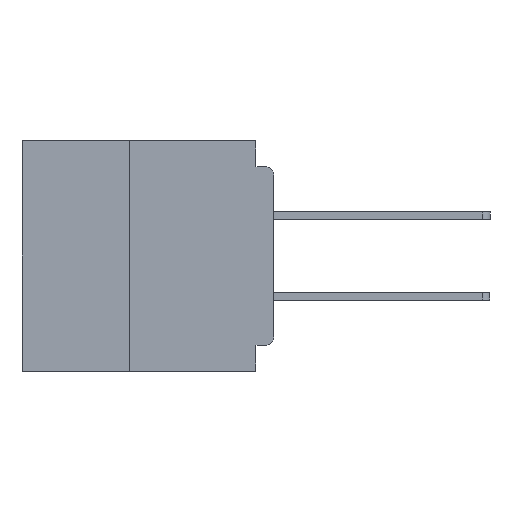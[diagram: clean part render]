
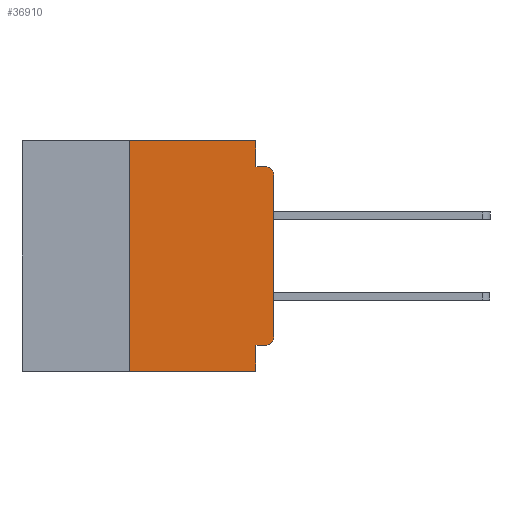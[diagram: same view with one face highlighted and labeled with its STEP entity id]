
A CAD part, left-side view. The second image highlights one B-rep face of the part: STEP entity #36910.
In plain terms, the highlighted planar face has unit normal (-1, 0, 0).
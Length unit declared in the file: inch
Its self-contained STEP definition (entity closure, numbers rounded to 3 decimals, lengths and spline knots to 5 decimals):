
#987 = CARTESIAN_POINT ( 'NONE',  ( 0., 0., -0.34 ) ) ;
#1331 = LINE ( 'NONE', #21667, #23645 ) ;
#1415 = EDGE_CURVE ( 'NONE', #28528, #23592, #11275, .T. ) ;
#1893 = ORIENTED_EDGE ( 'NONE', *, *, #25983, .F. ) ;
#2481 = VERTEX_POINT ( 'NONE', #31643 ) ;
#3035 = CARTESIAN_POINT ( 'NONE',  ( 0., 0., 0. ) ) ;
#3039 = CARTESIAN_POINT ( 'NONE',  ( 0., 0.25, -0.4 ) ) ;
#3169 = DIRECTION ( 'NONE',  ( 0., 0., 1. ) ) ;
#3193 = VECTOR ( 'NONE', #30604, 39.37008 ) ;
#3470 = EDGE_CURVE ( 'NONE', #35224, #23592, #12240, .T. ) ;
#3504 = CARTESIAN_POINT ( 'NONE',  ( 0., 0.015, -0.045 ) ) ;
#4850 = EDGE_CURVE ( 'NONE', #10057, #22910, #9841, .T. ) ;
#5433 = CARTESIAN_POINT ( 'NONE',  ( 0., 0.437, 0. ) ) ;
#5462 = EDGE_CURVE ( 'NONE', #35224, #2481, #33309, .T. ) ;
#6059 = DIRECTION ( 'NONE',  ( 0., 0., 1. ) ) ;
#7000 = CARTESIAN_POINT ( 'NONE',  ( 0., 0.437, -0.4 ) ) ;
#7153 = CARTESIAN_POINT ( 'NONE',  ( 0., 0.031, -0.4 ) ) ;
#7585 = LINE ( 'NONE', #32341, #38575 ) ;
#7809 = DIRECTION ( 'NONE',  ( -1., 0., 0. ) ) ;
#8521 = PLANE ( 'NONE',  #28601 ) ;
#9280 = VECTOR ( 'NONE', #3169, 39.37008 ) ;
#9346 = VECTOR ( 'NONE', #36983, 39.37008 ) ;
#9600 = CIRCLE ( 'NONE', #16299, 0.015 ) ;
#9841 = LINE ( 'NONE', #30610, #24982 ) ;
#9846 = DIRECTION ( 'NONE',  ( 0., -1., 0. ) ) ;
#10057 = VERTEX_POINT ( 'NONE', #24387 ) ;
#10333 = CARTESIAN_POINT ( 'NONE',  ( 0., 0.015, -0.355 ) ) ;
#11275 = LINE ( 'NONE', #13278, #3193 ) ;
#11592 = DIRECTION ( 'NONE',  ( 1., 0., 0. ) ) ;
#11731 = EDGE_CURVE ( 'NONE', #24256, #30757, #34052, .T. ) ;
#11870 = ORIENTED_EDGE ( 'NONE', *, *, #5462, .F. ) ;
#12240 = LINE ( 'NONE', #7000, #27360 ) ;
#13278 = CARTESIAN_POINT ( 'NONE',  ( 0., 0.031, -0.4 ) ) ;
#13606 = EDGE_CURVE ( 'NONE', #31149, #10057, #7585, .T. ) ;
#14590 = CARTESIAN_POINT ( 'NONE',  ( 0., 0.015, -0.34 ) ) ;
#15170 = ORIENTED_EDGE ( 'NONE', *, *, #4850, .F. ) ;
#15657 = ORIENTED_EDGE ( 'NONE', *, *, #11731, .T. ) ;
#16299 = AXIS2_PLACEMENT_3D ( 'NONE', #25949, #7809, #28965 ) ;
#17634 = DIRECTION ( 'NONE',  ( 0., 0., -1. ) ) ;
#18174 = VERTEX_POINT ( 'NONE', #38862 ) ;
#18314 = LINE ( 'NONE', #22138, #9346 ) ;
#18463 = FACE_OUTER_BOUND ( 'NONE', #36308, .T. ) ;
#19239 = VECTOR ( 'NONE', #6059, 39.37008 ) ;
#20994 = CARTESIAN_POINT ( 'NONE',  ( 0., 0.031, 0. ) ) ;
#21667 = CARTESIAN_POINT ( 'NONE',  ( 0., 0.437, 0. ) ) ;
#21884 = EDGE_CURVE ( 'NONE', #18174, #22910, #9600, .T. ) ;
#22124 = CARTESIAN_POINT ( 'NONE',  ( 0., 0.031, -0.355 ) ) ;
#22138 = CARTESIAN_POINT ( 'NONE',  ( 0., 0., -0.355 ) ) ;
#22910 = VERTEX_POINT ( 'NONE', #3504 ) ;
#23493 = DIRECTION ( 'NONE',  ( 0., 0., -1. ) ) ;
#23592 = VERTEX_POINT ( 'NONE', #7153 ) ;
#23645 = VECTOR ( 'NONE', #24742, 39.37008 ) ;
#24256 = VERTEX_POINT ( 'NONE', #10333 ) ;
#24387 = CARTESIAN_POINT ( 'NONE',  ( 0., 0.031, -0.045 ) ) ;
#24742 = DIRECTION ( 'NONE',  ( 0., -1., 0. ) ) ;
#24982 = VECTOR ( 'NONE', #30529, 39.37008 ) ;
#25126 = ORIENTED_EDGE ( 'NONE', *, *, #13606, .F. ) ;
#25949 = CARTESIAN_POINT ( 'NONE',  ( 0., 0.015, -0.06 ) ) ;
#25983 = EDGE_CURVE ( 'NONE', #2481, #31149, #1331, .T. ) ;
#27157 = EDGE_CURVE ( 'NONE', #30757, #18174, #27283, .T. ) ;
#27283 = LINE ( 'NONE', #3035, #19239 ) ;
#27360 = VECTOR ( 'NONE', #9846, 39.37008 ) ;
#27938 = ORIENTED_EDGE ( 'NONE', *, *, #3470, .T. ) ;
#28256 = CARTESIAN_POINT ( 'NONE',  ( 0., 0.25, -0.4 ) ) ;
#28528 = VERTEX_POINT ( 'NONE', #22124 ) ;
#28601 = AXIS2_PLACEMENT_3D ( 'NONE', #5433, #11592, #32616 ) ;
#28965 = DIRECTION ( 'NONE',  ( 0., 0., -1. ) ) ;
#30529 = DIRECTION ( 'NONE',  ( 0., -1., 0. ) ) ;
#30604 = DIRECTION ( 'NONE',  ( 0., 0., -1. ) ) ;
#30610 = CARTESIAN_POINT ( 'NONE',  ( 0., 0., -0.045 ) ) ;
#30724 = ORIENTED_EDGE ( 'NONE', *, *, #31879, .F. ) ;
#30757 = VERTEX_POINT ( 'NONE', #987 ) ;
#31149 = VERTEX_POINT ( 'NONE', #20994 ) ;
#31643 = CARTESIAN_POINT ( 'NONE',  ( 0., 0.25, 0. ) ) ;
#31879 = EDGE_CURVE ( 'NONE', #24256, #28528, #18314, .T. ) ;
#32341 = CARTESIAN_POINT ( 'NONE',  ( 0., 0.031, 0. ) ) ;
#32616 = DIRECTION ( 'NONE',  ( 0., 0., -1. ) ) ;
#33309 = LINE ( 'NONE', #3039, #9280 ) ;
#33890 = AXIS2_PLACEMENT_3D ( 'NONE', #14590, #35576, #17634 ) ;
#34052 = CIRCLE ( 'NONE', #33890, 0.015 ) ;
#35224 = VERTEX_POINT ( 'NONE', #28256 ) ;
#35576 = DIRECTION ( 'NONE',  ( -1., 0., 0. ) ) ;
#36275 = ORIENTED_EDGE ( 'NONE', *, *, #27157, .T. ) ;
#36308 = EDGE_LOOP ( 'NONE', ( #36275, #38133, #15170, #25126, #1893, #11870, #27938, #37684, #30724, #15657 ) ) ;
#36910 = ADVANCED_FACE ( 'NONE', ( #18463 ), #8521, .F. ) ;
#36983 = DIRECTION ( 'NONE',  ( 0., 1., 0. ) ) ;
#37684 = ORIENTED_EDGE ( 'NONE', *, *, #1415, .F. ) ;
#38133 = ORIENTED_EDGE ( 'NONE', *, *, #21884, .T. ) ;
#38575 = VECTOR ( 'NONE', #23493, 39.37008 ) ;
#38862 = CARTESIAN_POINT ( 'NONE',  ( 0., 0., -0.06 ) ) ;
